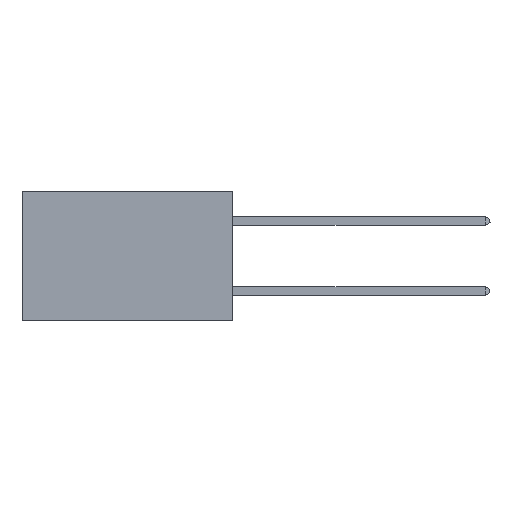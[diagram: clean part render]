
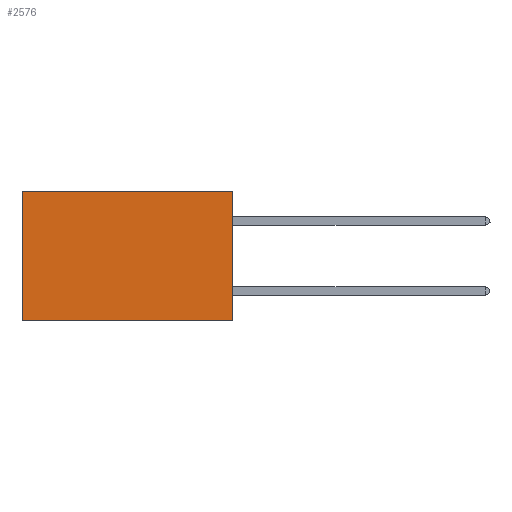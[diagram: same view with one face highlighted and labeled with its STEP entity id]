
A CAD part, left-side view. The second image highlights one B-rep face of the part: STEP entity #2576.
In plain terms, the highlighted planar face has unit normal (-1, 0, 0).
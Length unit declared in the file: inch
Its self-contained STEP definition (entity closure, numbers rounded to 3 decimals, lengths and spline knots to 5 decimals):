
#891 = CARTESIAN_POINT ( 'NONE',  ( 0.2875, 0., 0. ) ) ;
#1242 = CARTESIAN_POINT ( 'NONE',  ( 0.2875, 0.6, 0. ) ) ;
#2576 = ADVANCED_FACE ( 'NONE', ( #20618 ), #25454, .F. ) ;
#2844 = ORIENTED_EDGE ( 'NONE', *, *, #23608, .F. ) ;
#2905 = CARTESIAN_POINT ( 'NONE',  ( 0.2875, 0., 0. ) ) ;
#3599 = VECTOR ( 'NONE', #13036, 39.37008 ) ;
#3723 = CARTESIAN_POINT ( 'NONE',  ( 0.2875, 0., 0. ) ) ;
#4041 = DIRECTION ( 'NONE',  ( 0., 0., -1. ) ) ;
#4313 = LINE ( 'NONE', #1242, #12658 ) ;
#5706 = VERTEX_POINT ( 'NONE', #891 ) ;
#12658 = VECTOR ( 'NONE', #34907, 39.37008 ) ;
#12948 = EDGE_CURVE ( 'NONE', #20415, #30192, #4313, .T. ) ;
#13036 = DIRECTION ( 'NONE',  ( 0., 0., -1. ) ) ;
#13146 = CARTESIAN_POINT ( 'NONE',  ( 0.2875, 0., -0.37 ) ) ;
#13216 = VERTEX_POINT ( 'NONE', #36088 ) ;
#14085 = LINE ( 'NONE', #2905, #30225 ) ;
#14787 = AXIS2_PLACEMENT_3D ( 'NONE', #16428, #22531, #4041 ) ;
#15707 = ORIENTED_EDGE ( 'NONE', *, *, #12948, .T. ) ;
#16210 = DIRECTION ( 'NONE',  ( 0., 1., 0. ) ) ;
#16428 = CARTESIAN_POINT ( 'NONE',  ( 0.2875, 0., 0. ) ) ;
#16432 = ORIENTED_EDGE ( 'NONE', *, *, #31909, .T. ) ;
#16838 = VECTOR ( 'NONE', #16210, 39.37008 ) ;
#20415 = VERTEX_POINT ( 'NONE', #21824 ) ;
#20618 = FACE_OUTER_BOUND ( 'NONE', #25088, .T. ) ;
#21026 = LINE ( 'NONE', #3723, #3599 ) ;
#21430 = DIRECTION ( 'NONE',  ( 0., 1., 0. ) ) ;
#21824 = CARTESIAN_POINT ( 'NONE',  ( 0.2875, 0.6, 0. ) ) ;
#22531 = DIRECTION ( 'NONE',  ( 1., 0., 0. ) ) ;
#22575 = EDGE_CURVE ( 'NONE', #13216, #30192, #24908, .T. ) ;
#23608 = EDGE_CURVE ( 'NONE', #5706, #13216, #21026, .T. ) ;
#24908 = LINE ( 'NONE', #13146, #16838 ) ;
#25088 = EDGE_LOOP ( 'NONE', ( #15707, #37282, #2844, #16432 ) ) ;
#25454 = PLANE ( 'NONE',  #14787 ) ;
#30192 = VERTEX_POINT ( 'NONE', #34639 ) ;
#30225 = VECTOR ( 'NONE', #21430, 39.37008 ) ;
#31909 = EDGE_CURVE ( 'NONE', #5706, #20415, #14085, .T. ) ;
#34639 = CARTESIAN_POINT ( 'NONE',  ( 0.2875, 0.6, -0.37 ) ) ;
#34907 = DIRECTION ( 'NONE',  ( 0., 0., -1. ) ) ;
#36088 = CARTESIAN_POINT ( 'NONE',  ( 0.2875, 0., -0.37 ) ) ;
#37282 = ORIENTED_EDGE ( 'NONE', *, *, #22575, .F. ) ;
